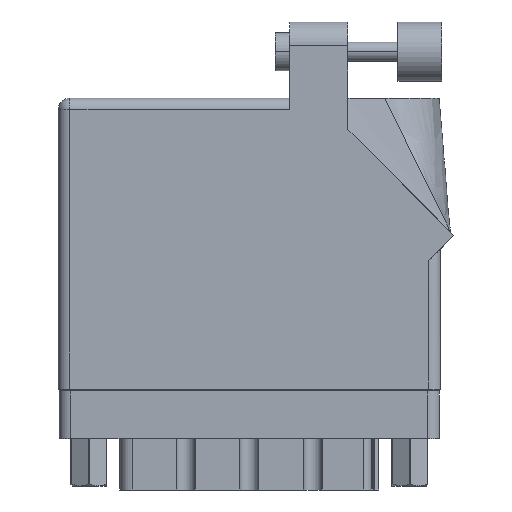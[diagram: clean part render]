
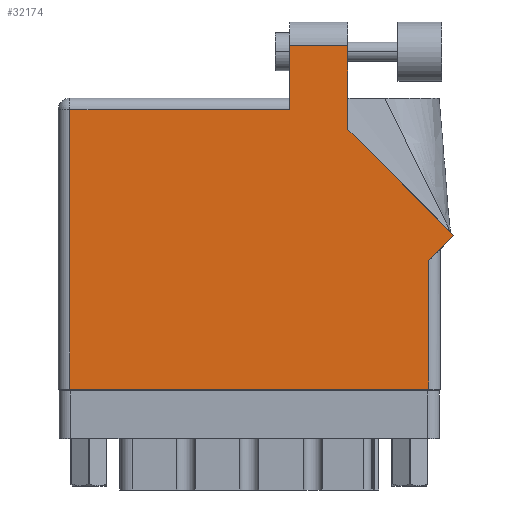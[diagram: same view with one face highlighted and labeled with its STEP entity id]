
A CAD part, front view. The second image highlights one B-rep face of the part: STEP entity #32174.
In plain terms, the highlighted face is planar.
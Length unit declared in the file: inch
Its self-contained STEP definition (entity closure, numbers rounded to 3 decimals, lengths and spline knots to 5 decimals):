
#378 = LINE ( 'NONE', #46643, #20741 ) ;
#1079 = DIRECTION ( 'NONE',  ( -1., 0., 0. ) ) ;
#1149 = VERTEX_POINT ( 'NONE', #44718 ) ;
#1597 = VECTOR ( 'NONE', #1079, 39.37008 ) ;
#1828 = DIRECTION ( 'NONE',  ( -1., 0., 0. ) ) ;
#1937 = CARTESIAN_POINT ( 'NONE',  ( 1.948, 0.737, 0. ) ) ;
#2330 = DIRECTION ( 'NONE',  ( 0., -1., 0. ) ) ;
#3226 = ORIENTED_EDGE ( 'NONE', *, *, #22312, .T. ) ;
#4471 = LINE ( 'NONE', #42162, #19612 ) ;
#4874 = DIRECTION ( 'NONE',  ( 0.707, 0.707, 0. ) ) ;
#7259 = DIRECTION ( 'NONE',  ( -0.707, 0.707, 0. ) ) ;
#8602 = CARTESIAN_POINT ( 'NONE',  ( 1.217, 1.805, 0. ) ) ;
#8885 = VERTEX_POINT ( 'NONE', #27814 ) ;
#9405 = LINE ( 'NONE', #21042, #37203 ) ;
#9412 = CARTESIAN_POINT ( 'NONE',  ( 0., 1.53, 0. ) ) ;
#10434 = VECTOR ( 'NONE', #44664, 39.37008 ) ;
#11692 = LINE ( 'NONE', #15973, #47637 ) ;
#12217 = VERTEX_POINT ( 'NONE', #41860 ) ;
#13638 = ORIENTED_EDGE ( 'NONE', *, *, #19526, .T. ) ;
#14111 = LINE ( 'NONE', #45470, #42354 ) ;
#15973 = CARTESIAN_POINT ( 'NONE',  ( 2.01, 0.737, 0. ) ) ;
#16794 = VECTOR ( 'NONE', #39319, 39.37008 ) ;
#16882 = VERTEX_POINT ( 'NONE', #8602 ) ;
#17546 = ORIENTED_EDGE ( 'NONE', *, *, #36632, .T. ) ;
#18708 = EDGE_CURVE ( 'NONE', #46606, #35618, #29769, .T. ) ;
#19102 = LINE ( 'NONE', #31012, #25792 ) ;
#19526 = EDGE_CURVE ( 'NONE', #35618, #12217, #11692, .T. ) ;
#19612 = VECTOR ( 'NONE', #31548, 39.37008 ) ;
#19668 = EDGE_CURVE ( 'NONE', #40962, #1149, #9405, .T. ) ;
#19709 = VERTEX_POINT ( 'NONE', #25341 ) ;
#20349 = EDGE_CURVE ( 'NONE', #12217, #8885, #19102, .T. ) ;
#20741 = VECTOR ( 'NONE', #43095, 39.37008 ) ;
#20890 = ORIENTED_EDGE ( 'NONE', *, *, #19668, .T. ) ;
#20946 = EDGE_CURVE ( 'NONE', #32968, #16882, #23850, .T. ) ;
#21042 = CARTESIAN_POINT ( 'NONE',  ( 0.062, 0., 0. ) ) ;
#21048 = DIRECTION ( 'NONE',  ( 0., 0., -1. ) ) ;
#21178 = CARTESIAN_POINT ( 'NONE',  ( 1.948, 0.675, 0. ) ) ;
#22312 = EDGE_CURVE ( 'NONE', #19709, #40962, #378, .T. ) ;
#22758 = ORIENTED_EDGE ( 'NONE', *, *, #20946, .T. ) ;
#23724 = CARTESIAN_POINT ( 'NONE',  ( 1.524, 1.805, 0. ) ) ;
#23847 = AXIS2_PLACEMENT_3D ( 'NONE', #9412, #21048, #1828 ) ;
#23850 = LINE ( 'NONE', #31948, #1597 ) ;
#24510 = ORIENTED_EDGE ( 'NONE', *, *, #20349, .T. ) ;
#25341 = CARTESIAN_POINT ( 'NONE',  ( 1.217, 1.468, 0. ) ) ;
#25606 = CARTESIAN_POINT ( 'NONE',  ( 0.062, 1.468, 0. ) ) ;
#25792 = VECTOR ( 'NONE', #7259, 39.37008 ) ;
#27691 = LINE ( 'NONE', #42871, #16794 ) ;
#27814 = CARTESIAN_POINT ( 'NONE',  ( 1.524, 1.36442, 0. ) ) ;
#29769 = LINE ( 'NONE', #1937, #10434 ) ;
#30764 = ORIENTED_EDGE ( 'NONE', *, *, #18708, .T. ) ;
#31012 = CARTESIAN_POINT ( 'NONE',  ( 2.08071, 0.80771, 0. ) ) ;
#31548 = DIRECTION ( 'NONE',  ( 1., 0., 0. ) ) ;
#31948 = CARTESIAN_POINT ( 'NONE',  ( 1.217, 1.805, 0. ) ) ;
#32174 = ADVANCED_FACE ( 'NONE', ( #47838 ), #48098, .F. ) ;
#32968 = VERTEX_POINT ( 'NONE', #23724 ) ;
#35618 = VERTEX_POINT ( 'NONE', #21178 ) ;
#36632 = EDGE_CURVE ( 'NONE', #1149, #46606, #4471, .T. ) ;
#37203 = VECTOR ( 'NONE', #2330, 39.37008 ) ;
#37229 = CARTESIAN_POINT ( 'NONE',  ( 1.948, 0., 0. ) ) ;
#37934 = EDGE_CURVE ( 'NONE', #8885, #32968, #14111, .T. ) ;
#38369 = ORIENTED_EDGE ( 'NONE', *, *, #37934, .T. ) ;
#39319 = DIRECTION ( 'NONE',  ( 0., -1., 0. ) ) ;
#40962 = VERTEX_POINT ( 'NONE', #25606 ) ;
#41860 = CARTESIAN_POINT ( 'NONE',  ( 2.08071, 0.80771, 0. ) ) ;
#42162 = CARTESIAN_POINT ( 'NONE',  ( 0., 0., 0. ) ) ;
#42354 = VECTOR ( 'NONE', #44978, 39.37008 ) ;
#42871 = CARTESIAN_POINT ( 'NONE',  ( 1.217, 1.53, 0. ) ) ;
#43095 = DIRECTION ( 'NONE',  ( -1., 0., 0. ) ) ;
#44664 = DIRECTION ( 'NONE',  ( 0., 1., 0. ) ) ;
#44718 = CARTESIAN_POINT ( 'NONE',  ( 0.062, 0., 0. ) ) ;
#44978 = DIRECTION ( 'NONE',  ( 0., 1., 0. ) ) ;
#45470 = CARTESIAN_POINT ( 'NONE',  ( 1.524, 1.36442, 0. ) ) ;
#45916 = ORIENTED_EDGE ( 'NONE', *, *, #49956, .T. ) ;
#46606 = VERTEX_POINT ( 'NONE', #37229 ) ;
#46643 = CARTESIAN_POINT ( 'NONE',  ( 0., 1.468, 0. ) ) ;
#47637 = VECTOR ( 'NONE', #4874, 39.37008 ) ;
#47838 = FACE_OUTER_BOUND ( 'NONE', #48734, .T. ) ;
#48098 = PLANE ( 'NONE',  #23847 ) ;
#48734 = EDGE_LOOP ( 'NONE', ( #38369, #22758, #45916, #3226, #20890, #17546, #30764, #13638, #24510 ) ) ;
#49956 = EDGE_CURVE ( 'NONE', #16882, #19709, #27691, .T. ) ;
